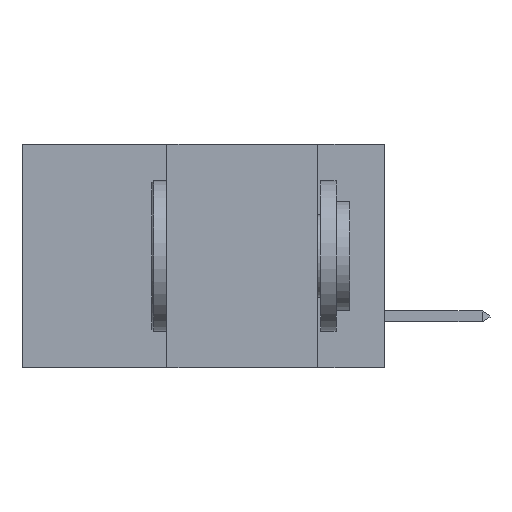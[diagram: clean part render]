
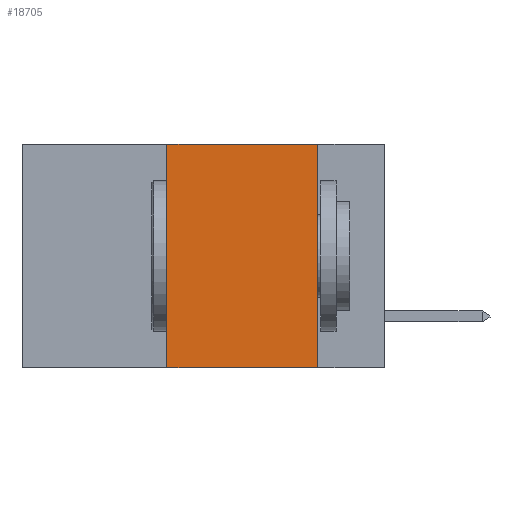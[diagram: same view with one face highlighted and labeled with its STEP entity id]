
A CAD part, left-side view. The second image highlights one B-rep face of the part: STEP entity #18705.
In plain terms, the highlighted planar face has unit normal (-1, 0, 0).
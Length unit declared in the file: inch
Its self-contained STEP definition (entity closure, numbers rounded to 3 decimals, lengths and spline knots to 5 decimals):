
#43 = VECTOR ( 'NONE', #4092, 39.37008 ) ;
#1225 = VERTEX_POINT ( 'NONE', #17080 ) ;
#1520 = VECTOR ( 'NONE', #6867, 39.37008 ) ;
#1938 = CARTESIAN_POINT ( 'NONE',  ( 0., 0.11, 0. ) ) ;
#2412 = PLANE ( 'NONE',  #3493 ) ;
#2588 = EDGE_CURVE ( 'NONE', #17812, #13766, #4953, .T. ) ;
#2851 = EDGE_CURVE ( 'NONE', #13766, #1225, #3680, .T. ) ;
#3180 = ORIENTED_EDGE ( 'NONE', *, *, #2851, .F. ) ;
#3209 = ORIENTED_EDGE ( 'NONE', *, *, #7557, .T. ) ;
#3493 = AXIS2_PLACEMENT_3D ( 'NONE', #13264, #16862, #9114 ) ;
#3680 = LINE ( 'NONE', #18072, #16889 ) ;
#4092 = DIRECTION ( 'NONE',  ( 0., 0., 1. ) ) ;
#4953 = LINE ( 'NONE', #11576, #1520 ) ;
#5210 = CARTESIAN_POINT ( 'NONE',  ( 0., 0.36, 0. ) ) ;
#5236 = EDGE_LOOP ( 'NONE', ( #3180, #10269, #13804, #3209 ) ) ;
#6867 = DIRECTION ( 'NONE',  ( 0., -1., 0. ) ) ;
#7557 = EDGE_CURVE ( 'NONE', #12460, #1225, #19702, .T. ) ;
#7829 = CARTESIAN_POINT ( 'NONE',  ( 0., 0.6, -0.37 ) ) ;
#9114 = DIRECTION ( 'NONE',  ( 0., 0., -1. ) ) ;
#10269 = ORIENTED_EDGE ( 'NONE', *, *, #2588, .F. ) ;
#10948 = FACE_OUTER_BOUND ( 'NONE', #5236, .T. ) ;
#11241 = LINE ( 'NONE', #14877, #43 ) ;
#11576 = CARTESIAN_POINT ( 'NONE',  ( 0., 0.6, 0. ) ) ;
#12406 = EDGE_CURVE ( 'NONE', #12460, #17812, #11241, .T. ) ;
#12460 = VERTEX_POINT ( 'NONE', #13436 ) ;
#13264 = CARTESIAN_POINT ( 'NONE',  ( 0., 0.6, 0. ) ) ;
#13436 = CARTESIAN_POINT ( 'NONE',  ( 0., 0.36, -0.37 ) ) ;
#13743 = DIRECTION ( 'NONE',  ( 0., -1., 0. ) ) ;
#13766 = VERTEX_POINT ( 'NONE', #1938 ) ;
#13804 = ORIENTED_EDGE ( 'NONE', *, *, #12406, .F. ) ;
#14877 = CARTESIAN_POINT ( 'NONE',  ( 0., 0.36, 0. ) ) ;
#14995 = DIRECTION ( 'NONE',  ( 0., 0., -1. ) ) ;
#15081 = VECTOR ( 'NONE', #13743, 39.37008 ) ;
#16862 = DIRECTION ( 'NONE',  ( 1., 0., 0. ) ) ;
#16889 = VECTOR ( 'NONE', #14995, 39.37008 ) ;
#17080 = CARTESIAN_POINT ( 'NONE',  ( 0., 0.11, -0.37 ) ) ;
#17812 = VERTEX_POINT ( 'NONE', #5210 ) ;
#18072 = CARTESIAN_POINT ( 'NONE',  ( 0., 0.11, 0. ) ) ;
#18705 = ADVANCED_FACE ( 'NONE', ( #10948 ), #2412, .F. ) ;
#19702 = LINE ( 'NONE', #7829, #15081 ) ;
